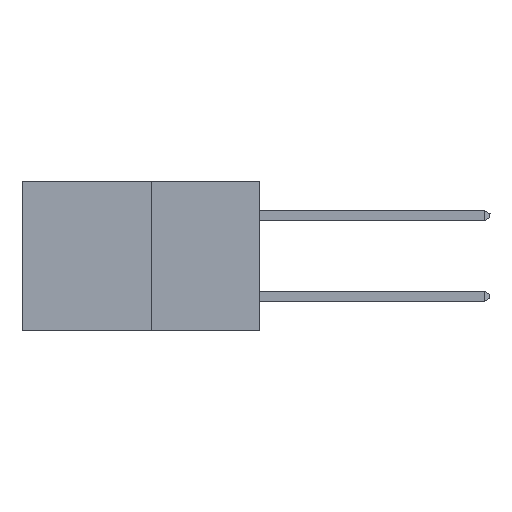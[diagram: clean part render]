
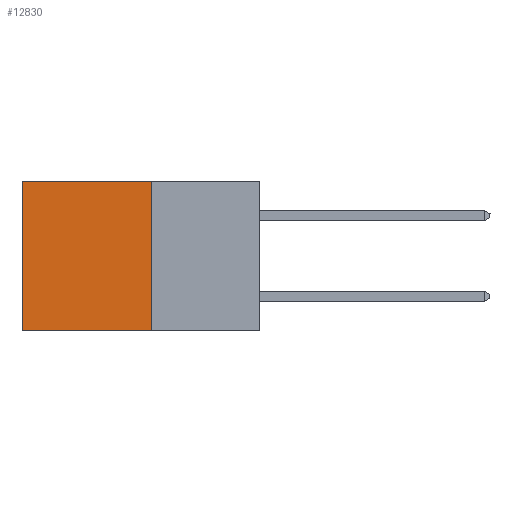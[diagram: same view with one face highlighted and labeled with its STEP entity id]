
A CAD part, left-side view. The second image highlights one B-rep face of the part: STEP entity #12830.
In plain terms, the highlighted planar face has unit normal (-1, 0, 0).
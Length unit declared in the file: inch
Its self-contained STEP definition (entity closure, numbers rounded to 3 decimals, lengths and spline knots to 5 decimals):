
#362 = ORIENTED_EDGE ( 'NONE', *, *, #3595, .F. ) ;
#2056 = DIRECTION ( 'NONE',  ( 0., 1., 0. ) ) ;
#2154 = CARTESIAN_POINT ( 'NONE',  ( 0.277, 0.27, 0. ) ) ;
#2567 = CARTESIAN_POINT ( 'NONE',  ( 0.277, 0.27, 0. ) ) ;
#3074 = CARTESIAN_POINT ( 'NONE',  ( 0.277, 0.27, -0.37 ) ) ;
#3319 = FACE_OUTER_BOUND ( 'NONE', #13645, .T. ) ;
#3376 = VECTOR ( 'NONE', #12689, 39.37008 ) ;
#3413 = PLANE ( 'NONE',  #7299 ) ;
#3595 = EDGE_CURVE ( 'NONE', #9296, #11420, #8779, .T. ) ;
#3995 = CARTESIAN_POINT ( 'NONE',  ( 0.277, 0.59, 0. ) ) ;
#4525 = DIRECTION ( 'NONE',  ( 1., 0., 0. ) ) ;
#4918 = DIRECTION ( 'NONE',  ( 0., 0., -1. ) ) ;
#4942 = CARTESIAN_POINT ( 'NONE',  ( 0.277, 0.59, -0.37 ) ) ;
#5022 = LINE ( 'NONE', #12723, #7860 ) ;
#5286 = EDGE_CURVE ( 'NONE', #9296, #13165, #9442, .T. ) ;
#5888 = LINE ( 'NONE', #12525, #11708 ) ;
#6052 = EDGE_CURVE ( 'NONE', #11420, #8117, #5022, .T. ) ;
#6546 = VECTOR ( 'NONE', #2056, 39.37008 ) ;
#7299 = AXIS2_PLACEMENT_3D ( 'NONE', #9906, #4525, #12140 ) ;
#7860 = VECTOR ( 'NONE', #12710, 39.37008 ) ;
#8117 = VERTEX_POINT ( 'NONE', #4942 ) ;
#8779 = LINE ( 'NONE', #12802, #3376 ) ;
#9137 = ORIENTED_EDGE ( 'NONE', *, *, #12420, .T. ) ;
#9296 = VERTEX_POINT ( 'NONE', #2567 ) ;
#9442 = LINE ( 'NONE', #2154, #6546 ) ;
#9547 = ORIENTED_EDGE ( 'NONE', *, *, #6052, .F. ) ;
#9906 = CARTESIAN_POINT ( 'NONE',  ( 0.277, 0.27, -0.37 ) ) ;
#11291 = ORIENTED_EDGE ( 'NONE', *, *, #5286, .T. ) ;
#11420 = VERTEX_POINT ( 'NONE', #3074 ) ;
#11708 = VECTOR ( 'NONE', #4918, 39.37008 ) ;
#12140 = DIRECTION ( 'NONE',  ( 0., 0., -1. ) ) ;
#12420 = EDGE_CURVE ( 'NONE', #13165, #8117, #5888, .T. ) ;
#12525 = CARTESIAN_POINT ( 'NONE',  ( 0.277, 0.59, -0.37 ) ) ;
#12689 = DIRECTION ( 'NONE',  ( 0., 0., -1. ) ) ;
#12710 = DIRECTION ( 'NONE',  ( 0., 1., 0. ) ) ;
#12723 = CARTESIAN_POINT ( 'NONE',  ( 0.277, 0.27, -0.37 ) ) ;
#12802 = CARTESIAN_POINT ( 'NONE',  ( 0.277, 0.27, -0.37 ) ) ;
#12830 = ADVANCED_FACE ( 'NONE', ( #3319 ), #3413, .F. ) ;
#13165 = VERTEX_POINT ( 'NONE', #3995 ) ;
#13645 = EDGE_LOOP ( 'NONE', ( #9137, #9547, #362, #11291 ) ) ;
